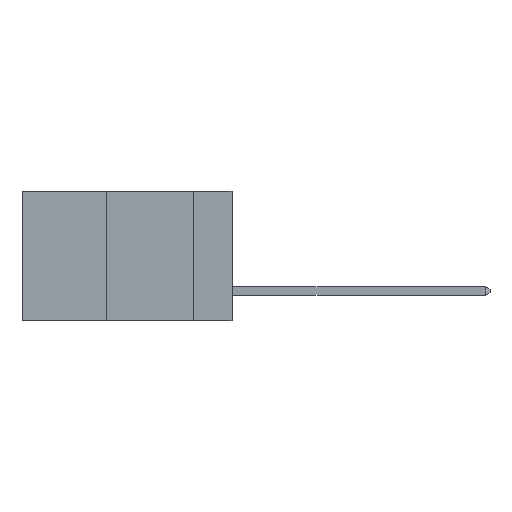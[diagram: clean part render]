
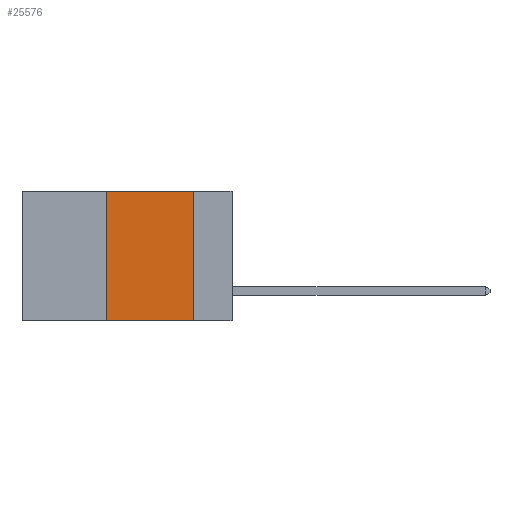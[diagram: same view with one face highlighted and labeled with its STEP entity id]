
A CAD part, left-side view. The second image highlights one B-rep face of the part: STEP entity #25576.
In plain terms, the highlighted planar face has unit normal (-1, 0, 0).
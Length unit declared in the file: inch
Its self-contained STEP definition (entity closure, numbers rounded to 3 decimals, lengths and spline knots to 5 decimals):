
#572 = CARTESIAN_POINT ( 'NONE',  ( 0., 0.36, 0. ) ) ;
#788 = CARTESIAN_POINT ( 'NONE',  ( 0., 0.36, 0. ) ) ;
#1262 = VERTEX_POINT ( 'NONE', #5131 ) ;
#2343 = FACE_OUTER_BOUND ( 'NONE', #23800, .T. ) ;
#2834 = LINE ( 'NONE', #26087, #11144 ) ;
#4807 = VECTOR ( 'NONE', #9986, 39.37008 ) ;
#5131 = CARTESIAN_POINT ( 'NONE',  ( 0., 0.11, 0. ) ) ;
#5370 = EDGE_CURVE ( 'NONE', #19314, #30415, #5796, .T. ) ;
#5796 = LINE ( 'NONE', #572, #4807 ) ;
#7507 = VECTOR ( 'NONE', #20224, 39.37008 ) ;
#7902 = ORIENTED_EDGE ( 'NONE', *, *, #5370, .F. ) ;
#7925 = CARTESIAN_POINT ( 'NONE',  ( 0., 0.11, 0. ) ) ;
#9986 = DIRECTION ( 'NONE',  ( 0., 0., 1. ) ) ;
#10188 = VERTEX_POINT ( 'NONE', #34434 ) ;
#11144 = VECTOR ( 'NONE', #13551, 39.37008 ) ;
#12286 = DIRECTION ( 'NONE',  ( 1., 0., 0. ) ) ;
#13551 = DIRECTION ( 'NONE',  ( 0., -1., 0. ) ) ;
#13897 = LINE ( 'NONE', #7925, #22200 ) ;
#15831 = LINE ( 'NONE', #35888, #7507 ) ;
#16394 = EDGE_CURVE ( 'NONE', #1262, #10188, #13897, .T. ) ;
#19314 = VERTEX_POINT ( 'NONE', #22661 ) ;
#20224 = DIRECTION ( 'NONE',  ( 0., -1., 0. ) ) ;
#21198 = EDGE_CURVE ( 'NONE', #30415, #1262, #15831, .T. ) ;
#22200 = VECTOR ( 'NONE', #29735, 39.37008 ) ;
#22661 = CARTESIAN_POINT ( 'NONE',  ( 0., 0.36, -0.37 ) ) ;
#23800 = EDGE_LOOP ( 'NONE', ( #25312, #37466, #7902, #31463 ) ) ;
#25312 = ORIENTED_EDGE ( 'NONE', *, *, #16394, .F. ) ;
#25576 = ADVANCED_FACE ( 'NONE', ( #2343 ), #40152, .F. ) ;
#26087 = CARTESIAN_POINT ( 'NONE',  ( 0., 0.6, -0.37 ) ) ;
#29735 = DIRECTION ( 'NONE',  ( 0., 0., -1. ) ) ;
#30415 = VERTEX_POINT ( 'NONE', #788 ) ;
#30965 = CARTESIAN_POINT ( 'NONE',  ( 0., 0.6, 0. ) ) ;
#31463 = ORIENTED_EDGE ( 'NONE', *, *, #33340, .T. ) ;
#31512 = AXIS2_PLACEMENT_3D ( 'NONE', #30965, #12286, #34083 ) ;
#33340 = EDGE_CURVE ( 'NONE', #19314, #10188, #2834, .T. ) ;
#34083 = DIRECTION ( 'NONE',  ( 0., 0., -1. ) ) ;
#34434 = CARTESIAN_POINT ( 'NONE',  ( 0., 0.11, -0.37 ) ) ;
#35888 = CARTESIAN_POINT ( 'NONE',  ( 0., 0.6, 0. ) ) ;
#37466 = ORIENTED_EDGE ( 'NONE', *, *, #21198, .F. ) ;
#40152 = PLANE ( 'NONE',  #31512 ) ;
